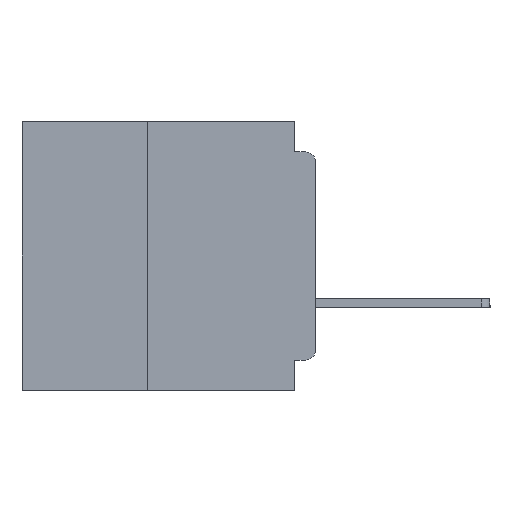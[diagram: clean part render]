
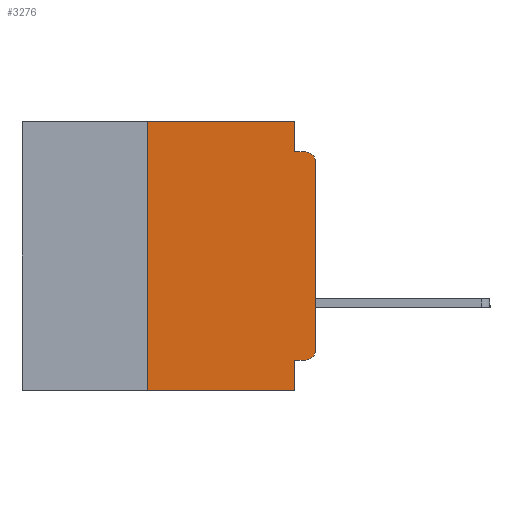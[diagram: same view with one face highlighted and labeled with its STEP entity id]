
A CAD part, left-side view. The second image highlights one B-rep face of the part: STEP entity #3276.
In plain terms, the highlighted planar face has unit normal (-1, 0, 0).
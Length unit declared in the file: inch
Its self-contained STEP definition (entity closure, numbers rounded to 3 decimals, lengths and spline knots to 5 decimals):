
#50 = ORIENTED_EDGE ( 'NONE', *, *, #44335, .T. ) ;
#1078 = ORIENTED_EDGE ( 'NONE', *, *, #42680, .F. ) ;
#2096 = VERTEX_POINT ( 'NONE', #34260 ) ;
#2560 = LINE ( 'NONE', #46217, #12028 ) ;
#2567 = LINE ( 'NONE', #40079, #9535 ) ;
#3153 = ORIENTED_EDGE ( 'NONE', *, *, #30203, .F. ) ;
#3195 = DIRECTION ( 'NONE',  ( 0., -1., 0. ) ) ;
#3276 = ADVANCED_FACE ( 'NONE', ( #41737 ), #37417, .F. ) ;
#3301 = CARTESIAN_POINT ( 'NONE',  ( 0., 0., -0.355 ) ) ;
#4411 = CARTESIAN_POINT ( 'NONE',  ( 0., 0., 0. ) ) ;
#4886 = LINE ( 'NONE', #50636, #23704 ) ;
#5587 = ORIENTED_EDGE ( 'NONE', *, *, #34129, .F. ) ;
#6288 = CARTESIAN_POINT ( 'NONE',  ( 0., 0.25, -0.4 ) ) ;
#6451 = VECTOR ( 'NONE', #40290, 39.37008 ) ;
#6600 = DIRECTION ( 'NONE',  ( 0., 0., -1. ) ) ;
#6765 = EDGE_CURVE ( 'NONE', #11038, #11452, #2560, .T. ) ;
#8258 = EDGE_CURVE ( 'NONE', #33843, #10330, #23895, .T. ) ;
#8662 = ORIENTED_EDGE ( 'NONE', *, *, #6765, .T. ) ;
#8817 = ORIENTED_EDGE ( 'NONE', *, *, #44110, .F. ) ;
#9535 = VECTOR ( 'NONE', #44061, 39.37008 ) ;
#10330 = VERTEX_POINT ( 'NONE', #17436 ) ;
#11038 = VERTEX_POINT ( 'NONE', #6288 ) ;
#11452 = VERTEX_POINT ( 'NONE', #12946 ) ;
#11601 = CARTESIAN_POINT ( 'NONE',  ( 0., 0.015, -0.355 ) ) ;
#11833 = ORIENTED_EDGE ( 'NONE', *, *, #15670, .T. ) ;
#12028 = VECTOR ( 'NONE', #26348, 39.37008 ) ;
#12362 = CARTESIAN_POINT ( 'NONE',  ( 0., 0.437, 0. ) ) ;
#12498 = VERTEX_POINT ( 'NONE', #11601 ) ;
#12946 = CARTESIAN_POINT ( 'NONE',  ( 0., 0.031, -0.4 ) ) ;
#13752 = CARTESIAN_POINT ( 'NONE',  ( 0., 0.031, -0.355 ) ) ;
#14799 = VERTEX_POINT ( 'NONE', #31021 ) ;
#15380 = CARTESIAN_POINT ( 'NONE',  ( 0., 0.031, -0.045 ) ) ;
#15670 = EDGE_CURVE ( 'NONE', #12498, #2096, #17049, .T. ) ;
#15840 = DIRECTION ( 'NONE',  ( -1., 0., 0. ) ) ;
#16426 = VERTEX_POINT ( 'NONE', #41592 ) ;
#16759 = ORIENTED_EDGE ( 'NONE', *, *, #24528, .F. ) ;
#17049 = CIRCLE ( 'NONE', #42723, 0.015 ) ;
#17082 = DIRECTION ( 'NONE',  ( -1., 0., 0. ) ) ;
#17136 = LINE ( 'NONE', #12362, #6451 ) ;
#17436 = CARTESIAN_POINT ( 'NONE',  ( 0., 0.015, -0.045 ) ) ;
#17656 = VECTOR ( 'NONE', #28420, 39.37008 ) ;
#17684 = LINE ( 'NONE', #3301, #37668 ) ;
#18315 = VECTOR ( 'NONE', #3195, 39.37008 ) ;
#18741 = CARTESIAN_POINT ( 'NONE',  ( 0., 0.031, -0.4 ) ) ;
#19730 = VECTOR ( 'NONE', #6600, 39.37008 ) ;
#21043 = VERTEX_POINT ( 'NONE', #15380 ) ;
#23143 = AXIS2_PLACEMENT_3D ( 'NONE', #39759, #15840, #43746 ) ;
#23704 = VECTOR ( 'NONE', #50800, 39.37008 ) ;
#23895 = CIRCLE ( 'NONE', #23143, 0.015 ) ;
#24528 = EDGE_CURVE ( 'NONE', #12498, #31594, #17684, .T. ) ;
#26348 = DIRECTION ( 'NONE',  ( 0., -1., 0. ) ) ;
#27222 = CARTESIAN_POINT ( 'NONE',  ( 0., 0., -0.045 ) ) ;
#27505 = DIRECTION ( 'NONE',  ( 0., 1., 0. ) ) ;
#28420 = DIRECTION ( 'NONE',  ( 0., 0., 1. ) ) ;
#30203 = EDGE_CURVE ( 'NONE', #16426, #21043, #2567, .T. ) ;
#31021 = CARTESIAN_POINT ( 'NONE',  ( 0., 0.25, 0. ) ) ;
#31440 = ORIENTED_EDGE ( 'NONE', *, *, #48113, .F. ) ;
#31594 = VERTEX_POINT ( 'NONE', #13752 ) ;
#32097 = EDGE_LOOP ( 'NONE', ( #50, #47597, #8817, #3153, #1078, #5587, #8662, #31440, #16759, #11833 ) ) ;
#33026 = AXIS2_PLACEMENT_3D ( 'NONE', #38893, #36446, #35698 ) ;
#33843 = VERTEX_POINT ( 'NONE', #40895 ) ;
#34129 = EDGE_CURVE ( 'NONE', #11038, #14799, #4886, .T. ) ;
#34260 = CARTESIAN_POINT ( 'NONE',  ( 0., 0., -0.34 ) ) ;
#35698 = DIRECTION ( 'NONE',  ( 0., 0., -1. ) ) ;
#36446 = DIRECTION ( 'NONE',  ( 1., 0., 0. ) ) ;
#37417 = PLANE ( 'NONE',  #33026 ) ;
#37668 = VECTOR ( 'NONE', #27505, 39.37008 ) ;
#38893 = CARTESIAN_POINT ( 'NONE',  ( 0., 0.437, 0. ) ) ;
#39759 = CARTESIAN_POINT ( 'NONE',  ( 0., 0.015, -0.06 ) ) ;
#40079 = CARTESIAN_POINT ( 'NONE',  ( 0., 0.031, 0. ) ) ;
#40290 = DIRECTION ( 'NONE',  ( 0., -1., 0. ) ) ;
#40895 = CARTESIAN_POINT ( 'NONE',  ( 0., 0., -0.06 ) ) ;
#40992 = CARTESIAN_POINT ( 'NONE',  ( 0., 0.015, -0.34 ) ) ;
#41592 = CARTESIAN_POINT ( 'NONE',  ( 0., 0.031, 0. ) ) ;
#41737 = FACE_OUTER_BOUND ( 'NONE', #32097, .T. ) ;
#42680 = EDGE_CURVE ( 'NONE', #14799, #16426, #17136, .T. ) ;
#42723 = AXIS2_PLACEMENT_3D ( 'NONE', #40992, #17082, #44992 ) ;
#43746 = DIRECTION ( 'NONE',  ( 0., 0., -1. ) ) ;
#44061 = DIRECTION ( 'NONE',  ( 0., 0., -1. ) ) ;
#44110 = EDGE_CURVE ( 'NONE', #21043, #10330, #50149, .T. ) ;
#44335 = EDGE_CURVE ( 'NONE', #2096, #33843, #50738, .T. ) ;
#44992 = DIRECTION ( 'NONE',  ( 0., 0., -1. ) ) ;
#46217 = CARTESIAN_POINT ( 'NONE',  ( 0., 0.437, -0.4 ) ) ;
#47597 = ORIENTED_EDGE ( 'NONE', *, *, #8258, .T. ) ;
#48113 = EDGE_CURVE ( 'NONE', #31594, #11452, #50302, .T. ) ;
#50149 = LINE ( 'NONE', #27222, #18315 ) ;
#50302 = LINE ( 'NONE', #18741, #19730 ) ;
#50636 = CARTESIAN_POINT ( 'NONE',  ( 0., 0.25, -0.4 ) ) ;
#50738 = LINE ( 'NONE', #4411, #17656 ) ;
#50800 = DIRECTION ( 'NONE',  ( 0., 0., 1. ) ) ;
